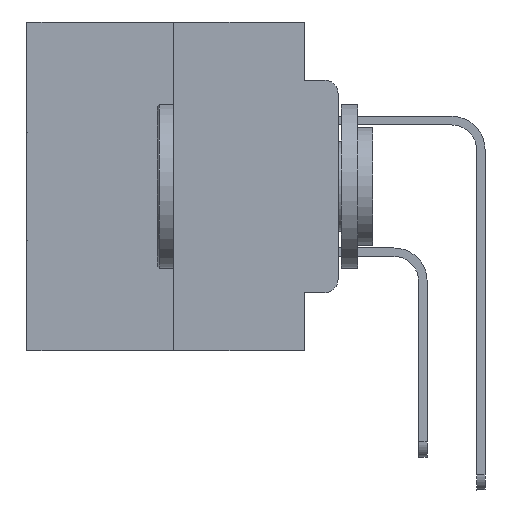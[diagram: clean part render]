
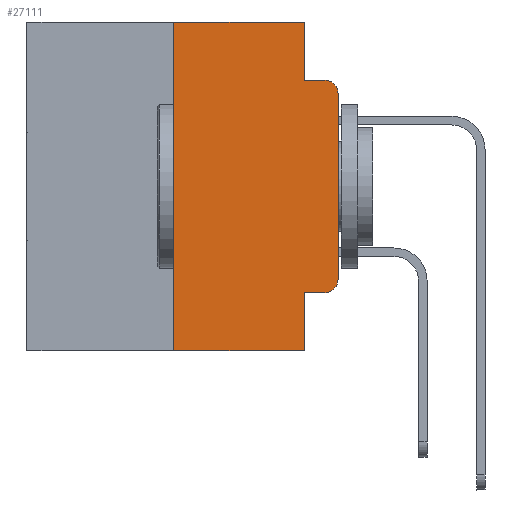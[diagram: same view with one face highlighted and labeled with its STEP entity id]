
A CAD part, left-side view. The second image highlights one B-rep face of the part: STEP entity #27111.
In plain terms, the highlighted planar face has unit normal (-1, 0, 0).
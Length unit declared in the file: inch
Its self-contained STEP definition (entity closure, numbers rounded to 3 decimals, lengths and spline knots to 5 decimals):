
#34 = LINE ( 'NONE', #4992, #31411 ) ;
#99 = DIRECTION ( 'NONE',  ( 1., 0., 0. ) ) ;
#138 = EDGE_CURVE ( 'NONE', #18928, #8263, #29293, .T. ) ;
#262 = CARTESIAN_POINT ( 'NONE',  ( 0., 0.473, 0. ) ) ;
#1484 = CARTESIAN_POINT ( 'NONE',  ( 0., 0.051, 0. ) ) ;
#1568 = ORIENTED_EDGE ( 'NONE', *, *, #25530, .T. ) ;
#1863 = VECTOR ( 'NONE', #2405, 39.37008 ) ;
#1873 = EDGE_CURVE ( 'NONE', #18928, #21038, #21455, .T. ) ;
#2295 = DIRECTION ( 'NONE',  ( 0., -1., 0. ) ) ;
#2405 = DIRECTION ( 'NONE',  ( 0., -1., 0. ) ) ;
#2747 = EDGE_CURVE ( 'NONE', #11029, #24026, #4850, .T. ) ;
#2969 = CARTESIAN_POINT ( 'NONE',  ( 0., 0.02, -0.4115 ) ) ;
#3296 = CARTESIAN_POINT ( 'NONE',  ( 0., 0.02, -0.3915 ) ) ;
#3497 = CARTESIAN_POINT ( 'NONE',  ( 0., 0.25, 0. ) ) ;
#3753 = VERTEX_POINT ( 'NONE', #29724 ) ;
#3830 = DIRECTION ( 'NONE',  ( 0., -1., 0. ) ) ;
#4642 = EDGE_CURVE ( 'NONE', #22551, #21038, #34, .T. ) ;
#4822 = CARTESIAN_POINT ( 'NONE',  ( 0., 0., 0. ) ) ;
#4850 = LINE ( 'NONE', #31427, #25263 ) ;
#4955 = EDGE_CURVE ( 'NONE', #8263, #3753, #7748, .T. ) ;
#4992 = CARTESIAN_POINT ( 'NONE',  ( 0., 0.473, -0.5 ) ) ;
#5049 = PLANE ( 'NONE',  #20466 ) ;
#6435 = LINE ( 'NONE', #1484, #22140 ) ;
#6550 = CARTESIAN_POINT ( 'NONE',  ( 0., 0.051, -0.0885 ) ) ;
#7725 = ORIENTED_EDGE ( 'NONE', *, *, #29980, .F. ) ;
#7748 = CIRCLE ( 'NONE', #18892, 0.02 ) ;
#8263 = VERTEX_POINT ( 'NONE', #2969 ) ;
#8536 = VERTEX_POINT ( 'NONE', #8844 ) ;
#8720 = DIRECTION ( 'NONE',  ( 0., 0., -1. ) ) ;
#8844 = CARTESIAN_POINT ( 'NONE',  ( 0., 0.051, -0.0885 ) ) ;
#9659 = ORIENTED_EDGE ( 'NONE', *, *, #1873, .F. ) ;
#9909 = EDGE_LOOP ( 'NONE', ( #18539, #1568, #10849, #7725, #10477, #21959, #17614, #9659, #30124, #26550 ) ) ;
#10477 = ORIENTED_EDGE ( 'NONE', *, *, #2747, .F. ) ;
#10517 = CARTESIAN_POINT ( 'NONE',  ( 0., 0.051, -0.4115 ) ) ;
#10759 = CIRCLE ( 'NONE', #26479, 0.02 ) ;
#10845 = LINE ( 'NONE', #6550, #23930 ) ;
#10849 = ORIENTED_EDGE ( 'NONE', *, *, #23941, .F. ) ;
#11029 = VERTEX_POINT ( 'NONE', #21793 ) ;
#12617 = LINE ( 'NONE', #3497, #25564 ) ;
#12729 = EDGE_CURVE ( 'NONE', #22551, #11029, #12617, .T. ) ;
#12923 = DIRECTION ( 'NONE',  ( 0., 0., 1. ) ) ;
#12948 = CARTESIAN_POINT ( 'NONE',  ( 0., 0.02, -0.0885 ) ) ;
#13505 = CARTESIAN_POINT ( 'NONE',  ( 0., 0.02, -0.1085 ) ) ;
#14961 = VECTOR ( 'NONE', #31177, 39.37008 ) ;
#15088 = DIRECTION ( 'NONE',  ( -1., 0., 0. ) ) ;
#16741 = LINE ( 'NONE', #4822, #25457 ) ;
#17126 = FACE_OUTER_BOUND ( 'NONE', #9909, .T. ) ;
#17614 = ORIENTED_EDGE ( 'NONE', *, *, #4642, .T. ) ;
#18539 = ORIENTED_EDGE ( 'NONE', *, *, #23541, .T. ) ;
#18832 = DIRECTION ( 'NONE',  ( 0., 0., -1. ) ) ;
#18892 = AXIS2_PLACEMENT_3D ( 'NONE', #3296, #15088, #22402 ) ;
#18928 = VERTEX_POINT ( 'NONE', #10517 ) ;
#19022 = VERTEX_POINT ( 'NONE', #30861 ) ;
#20342 = CARTESIAN_POINT ( 'NONE',  ( 0., 0.051, -0.5 ) ) ;
#20466 = AXIS2_PLACEMENT_3D ( 'NONE', #262, #99, #29395 ) ;
#21038 = VERTEX_POINT ( 'NONE', #20342 ) ;
#21455 = LINE ( 'NONE', #30703, #14961 ) ;
#21675 = DIRECTION ( 'NONE',  ( 0., 0., 1. ) ) ;
#21793 = CARTESIAN_POINT ( 'NONE',  ( 0., 0.25, 0. ) ) ;
#21959 = ORIENTED_EDGE ( 'NONE', *, *, #12729, .F. ) ;
#22140 = VECTOR ( 'NONE', #18832, 39.37008 ) ;
#22402 = DIRECTION ( 'NONE',  ( 0., 0., -1. ) ) ;
#22551 = VERTEX_POINT ( 'NONE', #28464 ) ;
#23541 = EDGE_CURVE ( 'NONE', #3753, #19022, #16741, .T. ) ;
#23930 = VECTOR ( 'NONE', #3830, 39.37008 ) ;
#23941 = EDGE_CURVE ( 'NONE', #8536, #29014, #10845, .T. ) ;
#24026 = VERTEX_POINT ( 'NONE', #28814 ) ;
#24202 = CARTESIAN_POINT ( 'NONE',  ( 0., 0.051, -0.4115 ) ) ;
#24711 = DIRECTION ( 'NONE',  ( 0., -1., 0. ) ) ;
#25263 = VECTOR ( 'NONE', #2295, 39.37008 ) ;
#25457 = VECTOR ( 'NONE', #21675, 39.37008 ) ;
#25530 = EDGE_CURVE ( 'NONE', #19022, #29014, #10759, .T. ) ;
#25564 = VECTOR ( 'NONE', #12923, 39.37008 ) ;
#25570 = DIRECTION ( 'NONE',  ( -1., 0., 0. ) ) ;
#26479 = AXIS2_PLACEMENT_3D ( 'NONE', #13505, #25570, #8720 ) ;
#26550 = ORIENTED_EDGE ( 'NONE', *, *, #4955, .T. ) ;
#27111 = ADVANCED_FACE ( 'NONE', ( #17126 ), #5049, .F. ) ;
#28464 = CARTESIAN_POINT ( 'NONE',  ( 0., 0.25, -0.5 ) ) ;
#28814 = CARTESIAN_POINT ( 'NONE',  ( 0., 0.051, 0. ) ) ;
#29014 = VERTEX_POINT ( 'NONE', #12948 ) ;
#29293 = LINE ( 'NONE', #24202, #1863 ) ;
#29395 = DIRECTION ( 'NONE',  ( 0., 0., -1. ) ) ;
#29724 = CARTESIAN_POINT ( 'NONE',  ( 0., 0., -0.3915 ) ) ;
#29980 = EDGE_CURVE ( 'NONE', #24026, #8536, #6435, .T. ) ;
#30124 = ORIENTED_EDGE ( 'NONE', *, *, #138, .T. ) ;
#30703 = CARTESIAN_POINT ( 'NONE',  ( 0., 0.051, 0. ) ) ;
#30861 = CARTESIAN_POINT ( 'NONE',  ( 0., 0., -0.1085 ) ) ;
#31177 = DIRECTION ( 'NONE',  ( 0., 0., -1. ) ) ;
#31411 = VECTOR ( 'NONE', #24711, 39.37008 ) ;
#31427 = CARTESIAN_POINT ( 'NONE',  ( 0., 0.473, 0. ) ) ;
